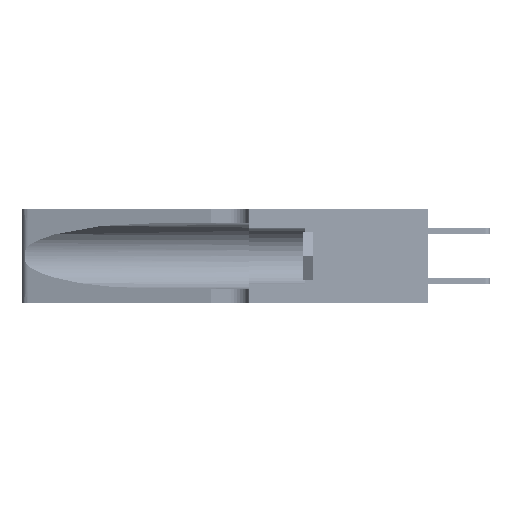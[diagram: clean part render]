
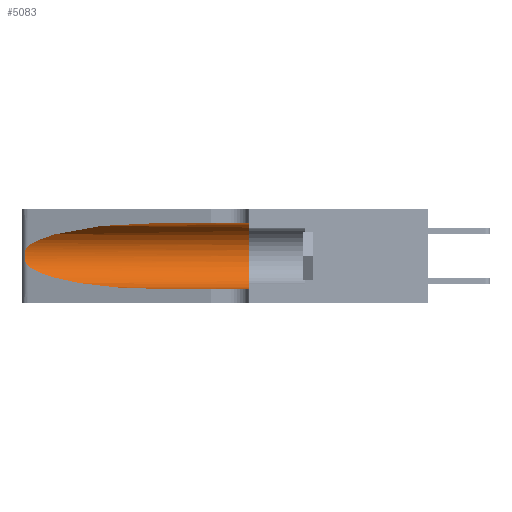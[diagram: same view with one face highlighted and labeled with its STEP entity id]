
A CAD part, left-side view. The second image highlights one B-rep face of the part: STEP entity #5083.
In plain terms, the highlighted cylindrical face has radius 3.308 mm (diameter 6.617 mm), a partial arc.
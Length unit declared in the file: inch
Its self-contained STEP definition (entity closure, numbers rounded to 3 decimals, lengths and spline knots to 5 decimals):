
#150 = CARTESIAN_POINT ( 'NONE',  ( 0.25856, 1.23593, 0.16098 ) ) ;
#269 = CARTESIAN_POINT ( 'NONE',  ( 0.26075, 1.23896, 0.178 ) ) ;
#309 = VERTEX_POINT ( 'NONE', #15625 ) ;
#2197 = CARTESIAN_POINT ( 'NONE',  ( 0.1305, 1.61858, 0.31525 ) ) ;
#2967 = EDGE_CURVE ( 'NONE', #8000, #8064, #39816, .T. ) ;
#3945 = CARTESIAN_POINT ( 'NONE',  ( 0.1305, 0.35, 0.31525 ) ) ;
#4040 = CARTESIAN_POINT ( 'NONE',  ( 0.25555, 1.22994, 0.2215 ) ) ;
#4845 = VERTEX_POINT ( 'NONE', #7976 ) ;
#4894 = CARTESIAN_POINT ( 'NONE',  ( 0.1305, 0.35, 0.05475 ) ) ;
#5083 = ADVANCED_FACE ( 'NONE', ( #32374 ), #28675, .F. ) ;
#6435 = CARTESIAN_POINT ( 'NONE',  ( 0.25487, 1.22718, 0.22369 ) ) ;
#6728 = CARTESIAN_POINT ( 'NONE',  ( 0.2373, 1.15595, 0.28018 ) ) ;
#6905 = DIRECTION ( 'NONE',  ( 0., 0., -1. ) ) ;
#6945 = ORIENTED_EDGE ( 'NONE', *, *, #28652, .T. ) ;
#7025 = VECTOR ( 'NONE', #42961, 39.37008 ) ;
#7500 = CARTESIAN_POINT ( 'NONE',  ( 0.25789, 1.23486, 0.15765 ) ) ;
#7976 = CARTESIAN_POINT ( 'NONE',  ( 0.1305, 0.72297, 0.31525 ) ) ;
#8000 = VERTEX_POINT ( 'NONE', #28938 ) ;
#8064 = VERTEX_POINT ( 'NONE', #13645 ) ;
#9365 = CARTESIAN_POINT ( 'NONE',  ( 0.2373, 1.15595, 0.08982 ) ) ;
#10056 = AXIS2_PLACEMENT_3D ( 'NONE', #16839, #37554, #6905 ) ;
#10084 = CARTESIAN_POINT ( 'NONE',  ( 0.18966, 0.96281, 0.31525 ) ) ;
#10543 = CARTESIAN_POINT ( 'NONE',  ( 0.25487, 1.22718, 0.22369 ) ) ;
#10582 = ORIENTED_EDGE ( 'NONE', *, *, #43201, .T. ) ;
#10828 = CARTESIAN_POINT ( 'NONE',  ( 0.25639, 1.23186, 0.15144 ) ) ;
#10964 = CARTESIAN_POINT ( 'NONE',  ( 0.25555, 1.22993, 0.14849 ) ) ;
#11166 = DIRECTION ( 'NONE',  ( 0., 1., 0. ) ) ;
#13261 = B_SPLINE_CURVE_WITH_KNOTS ( 'NONE', 3,
 ( #10543, #4040, #20573, #14250, #31132, #31274, #34694, #269, #41291, #150, #7500, #10828, #10964, #38113 ),
 .UNSPECIFIED., .F., .F.,
 ( 4, 2, 2, 2, 2, 2, 4 ),
 ( 0., 0.00027, 0.00053, 0.00107, 0.0016, 0.00187, 0.00214 ),
 .UNSPECIFIED. ) ;
#13645 = CARTESIAN_POINT ( 'NONE',  ( 0.1305, 0.72297, 0.05475 ) ) ;
#14250 = CARTESIAN_POINT ( 'NONE',  ( 0.25787, 1.23484, 0.2124 ) ) ;
#15625 = CARTESIAN_POINT ( 'NONE',  ( 0.25487, 1.22718, 0.22369 ) ) ;
#15680 = ORIENTED_EDGE ( 'NONE', *, *, #22596, .F. ) ;
#16575 =( BOUNDED_CURVE ( )  B_SPLINE_CURVE ( 3, ( #26954, #10084, #6728, #6435 ),
 .UNSPECIFIED., .F., .F. ) 
 B_SPLINE_CURVE_WITH_KNOTS ( ( 4, 4 ),
 ( 1.5708, 2.84003 ),
 .UNSPECIFIED. ) 
 CURVE ( )  GEOMETRIC_REPRESENTATION_ITEM ( )  RATIONAL_B_SPLINE_CURVE ( ( 1., 0.87, 0.87, 1. ) ) 
 REPRESENTATION_ITEM ( '' )  );
#16839 = CARTESIAN_POINT ( 'NONE',  ( 0.1305, 1.61858, 0.185 ) ) ;
#17355 = CIRCLE ( 'NONE', #30911, 0.13025 ) ;
#17596 = VERTEX_POINT ( 'NONE', #4894 ) ;
#18193 = DIRECTION ( 'NONE',  ( 0., 0., 1. ) ) ;
#19084 = CARTESIAN_POINT ( 'NONE',  ( 0.1305, 1.61858, 0.05475 ) ) ;
#19873 = DIRECTION ( 'NONE',  ( 0., -1., 0. ) ) ;
#20212 = VERTEX_POINT ( 'NONE', #3945 ) ;
#20573 = CARTESIAN_POINT ( 'NONE',  ( 0.25639, 1.23184, 0.21858 ) ) ;
#20819 = ORIENTED_EDGE ( 'NONE', *, *, #2967, .T. ) ;
#21837 = ORIENTED_EDGE ( 'NONE', *, *, #42638, .F. ) ;
#22596 = EDGE_CURVE ( 'NONE', #20212, #17596, #17355, .T. ) ;
#26954 = CARTESIAN_POINT ( 'NONE',  ( 0.1305, 0.72297, 0.31525 ) ) ;
#28652 = EDGE_CURVE ( 'NONE', #4845, #309, #16575, .T. ) ;
#28675 = CYLINDRICAL_SURFACE ( 'NONE', #10056, 0.13025 ) ;
#28938 = CARTESIAN_POINT ( 'NONE',  ( 0.25487, 1.22718, 0.14631 ) ) ;
#30086 = EDGE_CURVE ( 'NONE', #309, #8000, #13261, .T. ) ;
#30911 = AXIS2_PLACEMENT_3D ( 'NONE', #31633, #11166, #18193 ) ;
#31132 = CARTESIAN_POINT ( 'NONE',  ( 0.25854, 1.2359, 0.20912 ) ) ;
#31274 = CARTESIAN_POINT ( 'NONE',  ( 0.26018, 1.23835, 0.19895 ) ) ;
#31633 = CARTESIAN_POINT ( 'NONE',  ( 0.1305, 0.35, 0.185 ) ) ;
#32374 = FACE_OUTER_BOUND ( 'NONE', #34907, .T. ) ;
#34343 = LINE ( 'NONE', #2197, #44008 ) ;
#34694 = CARTESIAN_POINT ( 'NONE',  ( 0.26075, 1.23896, 0.19203 ) ) ;
#34802 = LINE ( 'NONE', #19084, #7025 ) ;
#34907 = EDGE_LOOP ( 'NONE', ( #6945, #39869, #20819, #10582, #15680, #21837 ) ) ;
#36678 = CARTESIAN_POINT ( 'NONE',  ( 0.18966, 0.96281, 0.05475 ) ) ;
#36971 = CARTESIAN_POINT ( 'NONE',  ( 0.25487, 1.22718, 0.14631 ) ) ;
#37554 = DIRECTION ( 'NONE',  ( 0., -1., 0. ) ) ;
#38113 = CARTESIAN_POINT ( 'NONE',  ( 0.25487, 1.22718, 0.14631 ) ) ;
#39816 =( BOUNDED_CURVE ( )  B_SPLINE_CURVE ( 3, ( #36971, #9365, #36678, #40113 ),
 .UNSPECIFIED., .F., .T. ) 
 B_SPLINE_CURVE_WITH_KNOTS ( ( 4, 4 ),
 ( 3.44316, 4.71239 ),
 .UNSPECIFIED. ) 
 CURVE ( )  GEOMETRIC_REPRESENTATION_ITEM ( )  RATIONAL_B_SPLINE_CURVE ( ( 1., 0.87, 0.87, 1. ) ) 
 REPRESENTATION_ITEM ( '' )  );
#39869 = ORIENTED_EDGE ( 'NONE', *, *, #30086, .T. ) ;
#40113 = CARTESIAN_POINT ( 'NONE',  ( 0.1305, 0.72297, 0.05475 ) ) ;
#41291 = CARTESIAN_POINT ( 'NONE',  ( 0.26017, 1.23833, 0.17102 ) ) ;
#42638 = EDGE_CURVE ( 'NONE', #4845, #20212, #34343, .T. ) ;
#42961 = DIRECTION ( 'NONE',  ( 0., -1., 0. ) ) ;
#43201 = EDGE_CURVE ( 'NONE', #8064, #17596, #34802, .T. ) ;
#44008 = VECTOR ( 'NONE', #19873, 39.37008 ) ;
